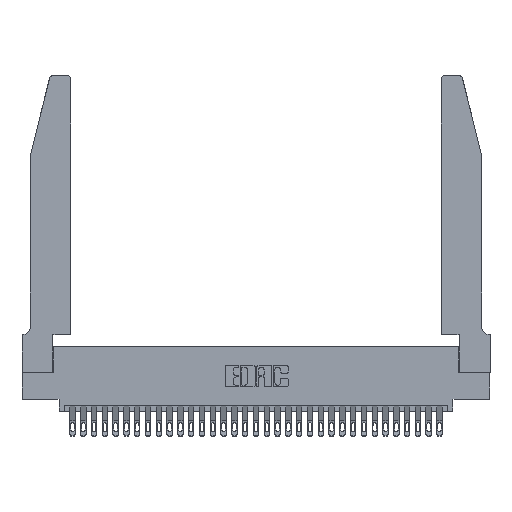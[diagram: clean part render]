
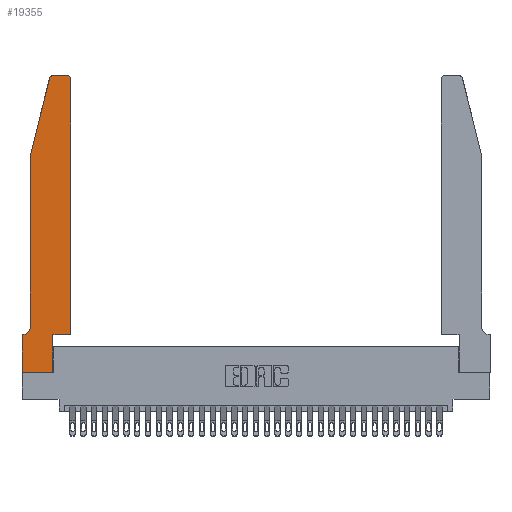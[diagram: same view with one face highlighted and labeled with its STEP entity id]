
A CAD part, top view. The second image highlights one B-rep face of the part: STEP entity #19355.
In plain terms, the highlighted planar face has unit normal (0, 0, 1).
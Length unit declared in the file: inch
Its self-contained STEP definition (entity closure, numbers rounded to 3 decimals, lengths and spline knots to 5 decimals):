
#636 = EDGE_CURVE ( 'NONE', #1610, #4503, #9847, .T. ) ;
#1387 = DIRECTION ( 'NONE',  ( -1., 0., 0. ) ) ;
#1610 = VERTEX_POINT ( 'NONE', #29006 ) ;
#1873 = EDGE_CURVE ( 'NONE', #32265, #28484, #33332, .T. ) ;
#1901 = DIRECTION ( 'NONE',  ( 0., 0., 1. ) ) ;
#2527 = ORIENTED_EDGE ( 'NONE', *, *, #25672, .T. ) ;
#3248 = CARTESIAN_POINT ( 'NONE',  ( 0.25487, 2.72718, 0.37 ) ) ;
#3482 = VERTEX_POINT ( 'NONE', #23476 ) ;
#3527 = EDGE_CURVE ( 'NONE', #3482, #18684, #29926, .T. ) ;
#3885 = ORIENTED_EDGE ( 'NONE', *, *, #20051, .T. ) ;
#4011 = EDGE_LOOP ( 'NONE', ( #13058, #33167, #3885, #21958, #22585, #16915, #30825, #15438, #12021, #2527, #4217, #9236 ) ) ;
#4108 = EDGE_CURVE ( 'NONE', #31659, #32265, #18476, .T. ) ;
#4217 = ORIENTED_EDGE ( 'NONE', *, *, #16799, .T. ) ;
#4357 = DIRECTION ( 'NONE',  ( 1., 0., 0. ) ) ;
#4503 = VERTEX_POINT ( 'NONE', #25664 ) ;
#4906 = DIRECTION ( 'NONE',  ( 0., 0., -1. ) ) ;
#4910 = LINE ( 'NONE', #22247, #31719 ) ;
#4967 = VECTOR ( 'NONE', #1387, 39.37008 ) ;
#6125 = LINE ( 'NONE', #22730, #31243 ) ;
#7057 = EDGE_CURVE ( 'NONE', #16572, #31659, #24849, .T. ) ;
#7149 = CARTESIAN_POINT ( 'NONE',  ( 0.0055, 0.35, 0.37 ) ) ;
#7483 = CARTESIAN_POINT ( 'NONE',  ( 0.0755, 2., 0.37 ) ) ;
#7886 = LINE ( 'NONE', #7993, #15561 ) ;
#7993 = CARTESIAN_POINT ( 'NONE',  ( 0.4505, 0.35, 0.37 ) ) ;
#8047 = DIRECTION ( 'NONE',  ( 0., 0., 1. ) ) ;
#8102 = EDGE_CURVE ( 'NONE', #18684, #18393, #22789, .T. ) ;
#8235 = VECTOR ( 'NONE', #20275, 39.37008 ) ;
#9236 = ORIENTED_EDGE ( 'NONE', *, *, #25125, .T. ) ;
#9391 = VECTOR ( 'NONE', #22539, 39.37008 ) ;
#9845 = CARTESIAN_POINT ( 'NONE',  ( 0.4205, 2.72, 0.37 ) ) ;
#9847 = LINE ( 'NONE', #33279, #8235 ) ;
#10074 = DIRECTION ( 'NONE',  ( 0., 1., 0. ) ) ;
#10269 = DIRECTION ( 'NONE',  ( 1., 0., 0. ) ) ;
#10405 = LINE ( 'NONE', #7483, #21687 ) ;
#10760 = AXIS2_PLACEMENT_3D ( 'NONE', #28650, #8047, #12796 ) ;
#11651 = VECTOR ( 'NONE', #29241, 39.37008 ) ;
#12021 = ORIENTED_EDGE ( 'NONE', *, *, #31739, .T. ) ;
#12293 = CIRCLE ( 'NONE', #15119, 0.07 ) ;
#12796 = DIRECTION ( 'NONE',  ( 1., 0., 0. ) ) ;
#12928 = VERTEX_POINT ( 'NONE', #15990 ) ;
#13058 = ORIENTED_EDGE ( 'NONE', *, *, #3527, .T. ) ;
#14679 = DIRECTION ( 'NONE',  ( -0.239, -0.971, 0. ) ) ;
#15119 = AXIS2_PLACEMENT_3D ( 'NONE', #20644, #4906, #25735 ) ;
#15438 = ORIENTED_EDGE ( 'NONE', *, *, #1873, .T. ) ;
#15445 = DIRECTION ( 'NONE',  ( 0., 1., 0. ) ) ;
#15561 = VECTOR ( 'NONE', #15445, 39.37008 ) ;
#15990 = CARTESIAN_POINT ( 'NONE',  ( 0.4505, 0.35, 0.37 ) ) ;
#16572 = VERTEX_POINT ( 'NONE', #7149 ) ;
#16799 = EDGE_CURVE ( 'NONE', #12928, #26992, #7886, .T. ) ;
#16915 = ORIENTED_EDGE ( 'NONE', *, *, #7057, .T. ) ;
#18393 = VERTEX_POINT ( 'NONE', #3248 ) ;
#18476 = LINE ( 'NONE', #23888, #11651 ) ;
#18684 = VERTEX_POINT ( 'NONE', #23550 ) ;
#19355 = ADVANCED_FACE ( 'NONE', ( #23794 ), #26010, .T. ) ;
#19762 = VECTOR ( 'NONE', #28381, 39.37008 ) ;
#19965 = CARTESIAN_POINT ( 'NONE',  ( 0., 0., 0.37 ) ) ;
#20051 = EDGE_CURVE ( 'NONE', #18393, #1610, #10405, .T. ) ;
#20124 = CARTESIAN_POINT ( 'NONE',  ( 0., 0.35, 0.37 ) ) ;
#20275 = DIRECTION ( 'NONE',  ( 0., -1., 0. ) ) ;
#20644 = CARTESIAN_POINT ( 'NONE',  ( 0.0055, 0.42, 0.37 ) ) ;
#21532 = EDGE_CURVE ( 'NONE', #4503, #16572, #12293, .T. ) ;
#21687 = VECTOR ( 'NONE', #14679, 39.37008 ) ;
#21958 = ORIENTED_EDGE ( 'NONE', *, *, #636, .T. ) ;
#22247 = CARTESIAN_POINT ( 'NONE',  ( 0.4505, 0.35, 0.37 ) ) ;
#22329 = AXIS2_PLACEMENT_3D ( 'NONE', #9845, #1901, #27961 ) ;
#22539 = DIRECTION ( 'NONE',  ( 1., 0., 0. ) ) ;
#22585 = ORIENTED_EDGE ( 'NONE', *, *, #21532, .T. ) ;
#22730 = CARTESIAN_POINT ( 'NONE',  ( 0.2865, 0.35, 0.37 ) ) ;
#22789 = CIRCLE ( 'NONE', #28917, 0.03 ) ;
#22972 = VERTEX_POINT ( 'NONE', #26998 ) ;
#23476 = CARTESIAN_POINT ( 'NONE',  ( 0.4205, 2.75, 0.37 ) ) ;
#23550 = CARTESIAN_POINT ( 'NONE',  ( 0.284, 2.75, 0.37 ) ) ;
#23794 = FACE_OUTER_BOUND ( 'NONE', #4011, .T. ) ;
#23888 = CARTESIAN_POINT ( 'NONE',  ( 0., 0., 0.37 ) ) ;
#24482 = CARTESIAN_POINT ( 'NONE',  ( 0., 0., 0.37 ) ) ;
#24849 = LINE ( 'NONE', #27803, #4967 ) ;
#25125 = EDGE_CURVE ( 'NONE', #26992, #3482, #28860, .T. ) ;
#25130 = CARTESIAN_POINT ( 'NONE',  ( 0.4505, 2.72, 0.37 ) ) ;
#25664 = CARTESIAN_POINT ( 'NONE',  ( 0.0755, 0.42, 0.37 ) ) ;
#25672 = EDGE_CURVE ( 'NONE', #22972, #12928, #4910, .T. ) ;
#25735 = DIRECTION ( 'NONE',  ( -1., 0., 0. ) ) ;
#25739 = CARTESIAN_POINT ( 'NONE',  ( 0.2605, 2.75, 0.37 ) ) ;
#26010 = PLANE ( 'NONE',  #10760 ) ;
#26159 = CARTESIAN_POINT ( 'NONE',  ( 0.2865, 0., 0.37 ) ) ;
#26992 = VERTEX_POINT ( 'NONE', #25130 ) ;
#26998 = CARTESIAN_POINT ( 'NONE',  ( 0.2865, 0.35, 0.37 ) ) ;
#27803 = CARTESIAN_POINT ( 'NONE',  ( 0.0755, 0.35, 0.37 ) ) ;
#27961 = DIRECTION ( 'NONE',  ( 1., 0., 0. ) ) ;
#28025 = DIRECTION ( 'NONE',  ( 0., 0., 1. ) ) ;
#28381 = DIRECTION ( 'NONE',  ( -1., 0., 0. ) ) ;
#28484 = VERTEX_POINT ( 'NONE', #26159 ) ;
#28650 = CARTESIAN_POINT ( 'NONE',  ( 0., 0.35, 0.37 ) ) ;
#28860 = CIRCLE ( 'NONE', #22329, 0.03 ) ;
#28917 = AXIS2_PLACEMENT_3D ( 'NONE', #30567, #28025, #10269 ) ;
#29006 = CARTESIAN_POINT ( 'NONE',  ( 0.0755, 2., 0.37 ) ) ;
#29241 = DIRECTION ( 'NONE',  ( 0., -1., 0. ) ) ;
#29926 = LINE ( 'NONE', #25739, #19762 ) ;
#30567 = CARTESIAN_POINT ( 'NONE',  ( 0.284, 2.72, 0.37 ) ) ;
#30825 = ORIENTED_EDGE ( 'NONE', *, *, #4108, .T. ) ;
#31243 = VECTOR ( 'NONE', #10074, 39.37008 ) ;
#31659 = VERTEX_POINT ( 'NONE', #20124 ) ;
#31719 = VECTOR ( 'NONE', #4357, 39.37008 ) ;
#31739 = EDGE_CURVE ( 'NONE', #28484, #22972, #6125, .T. ) ;
#32265 = VERTEX_POINT ( 'NONE', #19965 ) ;
#33167 = ORIENTED_EDGE ( 'NONE', *, *, #8102, .T. ) ;
#33279 = CARTESIAN_POINT ( 'NONE',  ( 0.0755, 2., 0.37 ) ) ;
#33332 = LINE ( 'NONE', #24482, #9391 ) ;
